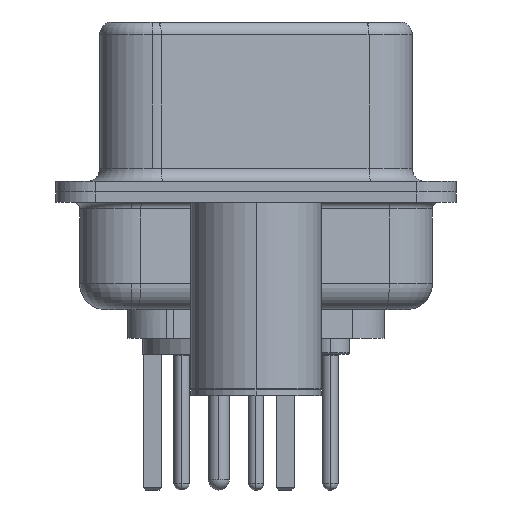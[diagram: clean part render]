
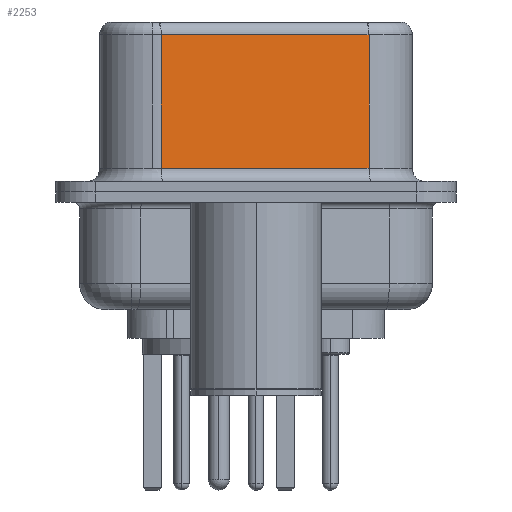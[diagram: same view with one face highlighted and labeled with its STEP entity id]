
A CAD part, left-side view. The second image highlights one B-rep face of the part: STEP entity #2253.
In plain terms, the highlighted planar face has unit normal (-0.985, -0.174, 0).
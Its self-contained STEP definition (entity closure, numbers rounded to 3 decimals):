
#1409 = ORIENTED_EDGE ( 'NONE', *, *, #31222, .T. ) ;
#2253 = ADVANCED_FACE ( 'NONE', ( #11705 ), #28610, .F. ) ;
#3314 = CARTESIAN_POINT ( 'NONE',  ( 5.132, -4.322, 0.9 ) ) ;
#3420 = DIRECTION ( 'NONE',  ( 0.174, -0.985, 0. ) ) ;
#4322 = CARTESIAN_POINT ( 'NONE',  ( 5.132, -4.322, 6.02 ) ) ;
#4537 = LINE ( 'NONE', #18336, #30861 ) ;
#4641 = LINE ( 'NONE', #33166, #12216 ) ;
#5403 = CARTESIAN_POINT ( 'NONE',  ( 3.73, 3.628, 0.9 ) ) ;
#5809 = VERTEX_POINT ( 'NONE', #25365 ) ;
#8168 = DIRECTION ( 'NONE',  ( 0., 0., -1. ) ) ;
#8524 = AXIS2_PLACEMENT_3D ( 'NONE', #11065, #25832, #33029 ) ;
#9649 = EDGE_LOOP ( 'NONE', ( #26698, #18505, #1409, #23692 ) ) ;
#10800 = VECTOR ( 'NONE', #3420, 1000. ) ;
#11065 = CARTESIAN_POINT ( 'NONE',  ( 5.132, -4.322, 6.52 ) ) ;
#11481 = CARTESIAN_POINT ( 'NONE',  ( 5.132, -4.322, 0.9 ) ) ;
#11705 = FACE_OUTER_BOUND ( 'NONE', #9649, .T. ) ;
#12216 = VECTOR ( 'NONE', #25557, 1000. ) ;
#13694 = EDGE_CURVE ( 'NONE', #21410, #16580, #26008, .T. ) ;
#16580 = VERTEX_POINT ( 'NONE', #11481 ) ;
#16743 = EDGE_CURVE ( 'NONE', #24598, #5809, #27522, .T. ) ;
#18336 = CARTESIAN_POINT ( 'NONE',  ( 3.73, 3.628, 6.52 ) ) ;
#18505 = ORIENTED_EDGE ( 'NONE', *, *, #16743, .T. ) ;
#18810 = EDGE_CURVE ( 'NONE', #24598, #16580, #4641, .T. ) ;
#21410 = VERTEX_POINT ( 'NONE', #5403 ) ;
#23692 = ORIENTED_EDGE ( 'NONE', *, *, #13694, .T. ) ;
#24598 = VERTEX_POINT ( 'NONE', #28532 ) ;
#25365 = CARTESIAN_POINT ( 'NONE',  ( 3.73, 3.628, 6.02 ) ) ;
#25557 = DIRECTION ( 'NONE',  ( 0., 0., -1. ) ) ;
#25832 = DIRECTION ( 'NONE',  ( 0.985, 0.174, 0. ) ) ;
#26008 = LINE ( 'NONE', #3314, #10800 ) ;
#26698 = ORIENTED_EDGE ( 'NONE', *, *, #18810, .F. ) ;
#26744 = VECTOR ( 'NONE', #29835, 1000. ) ;
#27522 = LINE ( 'NONE', #4322, #26744 ) ;
#28532 = CARTESIAN_POINT ( 'NONE',  ( 5.132, -4.322, 6.02 ) ) ;
#28610 = PLANE ( 'NONE',  #8524 ) ;
#29835 = DIRECTION ( 'NONE',  ( -0.174, 0.985, 0. ) ) ;
#30861 = VECTOR ( 'NONE', #8168, 1000. ) ;
#31222 = EDGE_CURVE ( 'NONE', #5809, #21410, #4537, .T. ) ;
#33029 = DIRECTION ( 'NONE',  ( -0.174, 0.985, 0. ) ) ;
#33166 = CARTESIAN_POINT ( 'NONE',  ( 5.132, -4.322, 6.52 ) ) ;
